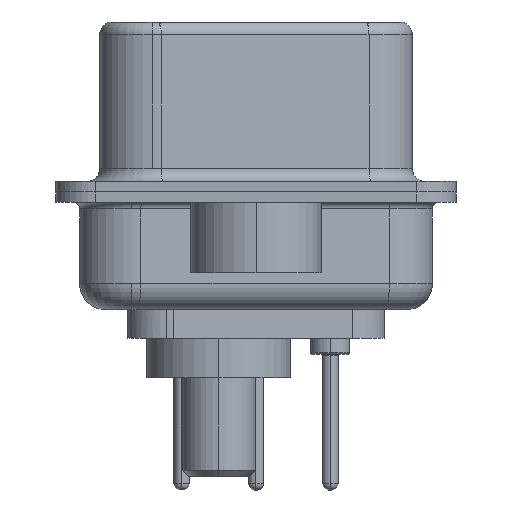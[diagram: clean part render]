
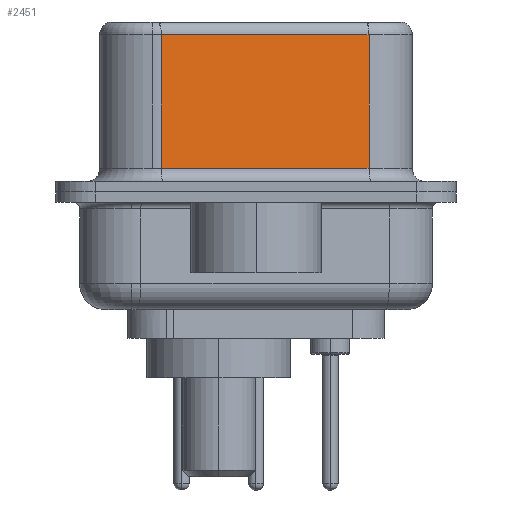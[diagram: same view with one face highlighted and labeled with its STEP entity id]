
A CAD part, left-side view. The second image highlights one B-rep face of the part: STEP entity #2451.
In plain terms, the highlighted planar face has unit normal (-0.985, -0.174, 0).
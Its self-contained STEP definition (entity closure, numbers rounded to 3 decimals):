
#636 = CARTESIAN_POINT ( 'NONE',  ( 3.73, 3.628, 6.02 ) ) ;
#819 = DIRECTION ( 'NONE',  ( 0., 0., -1. ) ) ;
#2451 = ADVANCED_FACE ( 'NONE', ( #12251 ), #20174, .F. ) ;
#2593 = CARTESIAN_POINT ( 'NONE',  ( 5.132, -4.322, 6.02 ) ) ;
#3615 = EDGE_CURVE ( 'NONE', #4588, #8675, #7295, .T. ) ;
#4317 = EDGE_CURVE ( 'NONE', #8675, #14359, #26450, .T. ) ;
#4588 = VERTEX_POINT ( 'NONE', #636 ) ;
#6801 = VECTOR ( 'NONE', #25759, 1000. ) ;
#7295 = LINE ( 'NONE', #15482, #12205 ) ;
#8675 = VERTEX_POINT ( 'NONE', #10451 ) ;
#9252 = EDGE_CURVE ( 'NONE', #11563, #4588, #25949, .T. ) ;
#10451 = CARTESIAN_POINT ( 'NONE',  ( 3.73, 3.628, 0.9 ) ) ;
#11230 = DIRECTION ( 'NONE',  ( 0.174, -0.985, 0. ) ) ;
#11563 = VERTEX_POINT ( 'NONE', #25269 ) ;
#11727 = LINE ( 'NONE', #13638, #6801 ) ;
#12205 = VECTOR ( 'NONE', #819, 1000. ) ;
#12251 = FACE_OUTER_BOUND ( 'NONE', #24547, .T. ) ;
#13638 = CARTESIAN_POINT ( 'NONE',  ( 5.132, -4.322, 6.52 ) ) ;
#13679 = CARTESIAN_POINT ( 'NONE',  ( 5.132, -4.322, 6.52 ) ) ;
#14119 = DIRECTION ( 'NONE',  ( -0.174, 0.985, 0. ) ) ;
#14359 = VERTEX_POINT ( 'NONE', #24087 ) ;
#14762 = DIRECTION ( 'NONE',  ( 0.985, 0.174, 0. ) ) ;
#15184 = VECTOR ( 'NONE', #16030, 1000. ) ;
#15482 = CARTESIAN_POINT ( 'NONE',  ( 3.73, 3.628, 6.52 ) ) ;
#15771 = EDGE_CURVE ( 'NONE', #11563, #14359, #11727, .T. ) ;
#16030 = DIRECTION ( 'NONE',  ( -0.174, 0.985, 0. ) ) ;
#17035 = ORIENTED_EDGE ( 'NONE', *, *, #3615, .T. ) ;
#17818 = ORIENTED_EDGE ( 'NONE', *, *, #4317, .T. ) ;
#20168 = ORIENTED_EDGE ( 'NONE', *, *, #15771, .F. ) ;
#20174 = PLANE ( 'NONE',  #20484 ) ;
#20484 = AXIS2_PLACEMENT_3D ( 'NONE', #13679, #14762, #14119 ) ;
#24087 = CARTESIAN_POINT ( 'NONE',  ( 5.132, -4.322, 0.9 ) ) ;
#24547 = EDGE_LOOP ( 'NONE', ( #20168, #25166, #17035, #17818 ) ) ;
#25166 = ORIENTED_EDGE ( 'NONE', *, *, #9252, .T. ) ;
#25201 = VECTOR ( 'NONE', #11230, 1000. ) ;
#25269 = CARTESIAN_POINT ( 'NONE',  ( 5.132, -4.322, 6.02 ) ) ;
#25759 = DIRECTION ( 'NONE',  ( 0., 0., -1. ) ) ;
#25949 = LINE ( 'NONE', #2593, #15184 ) ;
#26090 = CARTESIAN_POINT ( 'NONE',  ( 5.132, -4.322, 0.9 ) ) ;
#26450 = LINE ( 'NONE', #26090, #25201 ) ;
